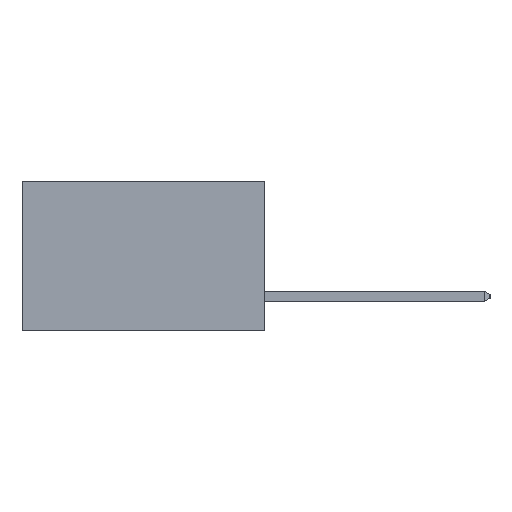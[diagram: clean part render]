
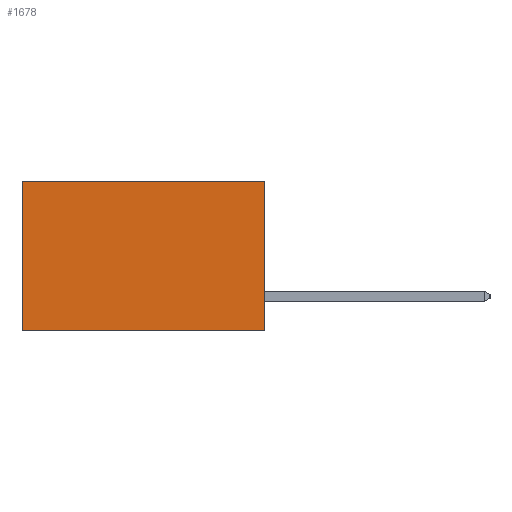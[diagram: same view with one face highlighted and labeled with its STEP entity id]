
A CAD part, left-side view. The second image highlights one B-rep face of the part: STEP entity #1678.
In plain terms, the highlighted planar face has unit normal (-1, 0, 0).
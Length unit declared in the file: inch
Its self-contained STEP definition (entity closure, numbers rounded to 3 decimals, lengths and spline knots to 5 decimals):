
#652 = DIRECTION ( 'NONE',  ( 0., 0., -1. ) ) ;
#939 = VECTOR ( 'NONE', #10885, 39.37008 ) ;
#965 = VERTEX_POINT ( 'NONE', #3164 ) ;
#1090 = DIRECTION ( 'NONE',  ( 0., 1., 0. ) ) ;
#1098 = ORIENTED_EDGE ( 'NONE', *, *, #2530, .F. ) ;
#1345 = DIRECTION ( 'NONE',  ( 0., 0., -1. ) ) ;
#1418 = EDGE_CURVE ( 'NONE', #4155, #10511, #4080, .T. ) ;
#1425 = DIRECTION ( 'NONE',  ( 1., 0., 0. ) ) ;
#1672 = CARTESIAN_POINT ( 'NONE',  ( 0.2615, 0., -0.37 ) ) ;
#1678 = ADVANCED_FACE ( 'NONE', ( #6788 ), #1753, .F. ) ;
#1753 = PLANE ( 'NONE',  #7774 ) ;
#1983 = EDGE_CURVE ( 'NONE', #965, #10511, #7964, .T. ) ;
#2134 = CARTESIAN_POINT ( 'NONE',  ( 0.2615, 0., -0.37 ) ) ;
#2530 = EDGE_CURVE ( 'NONE', #11058, #965, #4813, .T. ) ;
#2698 = VECTOR ( 'NONE', #652, 39.37008 ) ;
#3164 = CARTESIAN_POINT ( 'NONE',  ( 0.2615, 0., -0.37 ) ) ;
#3941 = ORIENTED_EDGE ( 'NONE', *, *, #8867, .T. ) ;
#3962 = CARTESIAN_POINT ( 'NONE',  ( 0.2615, 0.6, -0.37 ) ) ;
#4080 = LINE ( 'NONE', #6011, #10606 ) ;
#4155 = VERTEX_POINT ( 'NONE', #7877 ) ;
#4447 = LINE ( 'NONE', #9147, #10950 ) ;
#4813 = LINE ( 'NONE', #1672, #2698 ) ;
#5086 = EDGE_LOOP ( 'NONE', ( #8071, #10213, #1098, #3941 ) ) ;
#6011 = CARTESIAN_POINT ( 'NONE',  ( 0.2615, 0.6, -0.37 ) ) ;
#6135 = DIRECTION ( 'NONE',  ( 0., 0., -1. ) ) ;
#6788 = FACE_OUTER_BOUND ( 'NONE', #5086, .T. ) ;
#7639 = CARTESIAN_POINT ( 'NONE',  ( 0.2615, 0., 0. ) ) ;
#7774 = AXIS2_PLACEMENT_3D ( 'NONE', #2134, #1425, #1345 ) ;
#7877 = CARTESIAN_POINT ( 'NONE',  ( 0.2615, 0.6, 0. ) ) ;
#7964 = LINE ( 'NONE', #9200, #939 ) ;
#8071 = ORIENTED_EDGE ( 'NONE', *, *, #1418, .T. ) ;
#8867 = EDGE_CURVE ( 'NONE', #11058, #4155, #4447, .T. ) ;
#9147 = CARTESIAN_POINT ( 'NONE',  ( 0.2615, 0., 0. ) ) ;
#9200 = CARTESIAN_POINT ( 'NONE',  ( 0.2615, 0., -0.37 ) ) ;
#10213 = ORIENTED_EDGE ( 'NONE', *, *, #1983, .F. ) ;
#10511 = VERTEX_POINT ( 'NONE', #3962 ) ;
#10606 = VECTOR ( 'NONE', #6135, 39.37008 ) ;
#10885 = DIRECTION ( 'NONE',  ( 0., 1., 0. ) ) ;
#10950 = VECTOR ( 'NONE', #1090, 39.37008 ) ;
#11058 = VERTEX_POINT ( 'NONE', #7639 ) ;
